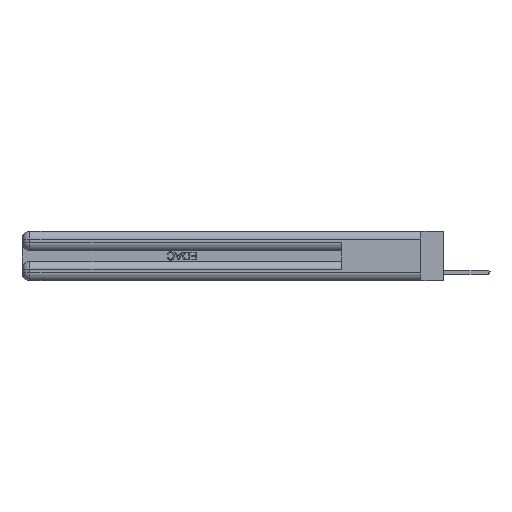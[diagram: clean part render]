
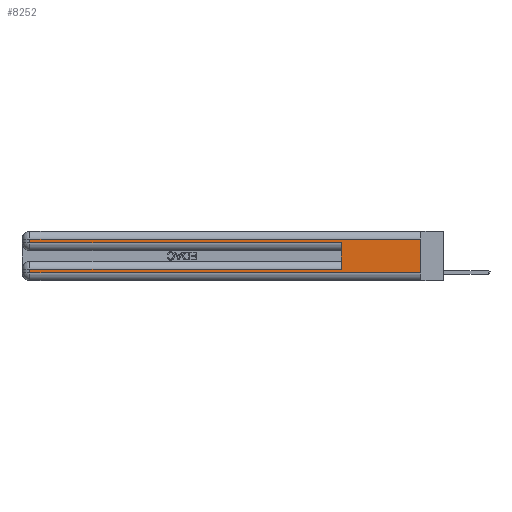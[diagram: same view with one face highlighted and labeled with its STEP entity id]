
A CAD part, left-side view. The second image highlights one B-rep face of the part: STEP entity #8252.
In plain terms, the highlighted planar face has unit normal (-1, 0, 0).
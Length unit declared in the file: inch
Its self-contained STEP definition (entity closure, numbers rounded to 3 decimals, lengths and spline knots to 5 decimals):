
#63 = VECTOR ( 'NONE', #7379, 39.37008 ) ;
#2607 = VECTOR ( 'NONE', #17444, 39.37008 ) ;
#3861 = CARTESIAN_POINT ( 'NONE',  ( 0., 0., 0.06 ) ) ;
#4646 = VECTOR ( 'NONE', #30315, 39.37008 ) ;
#4804 = DIRECTION ( 'NONE',  ( 0., 0., -1. ) ) ;
#5010 = PLANE ( 'NONE',  #29456 ) ;
#5038 = DIRECTION ( 'NONE',  ( 0., 1., 0. ) ) ;
#5150 = EDGE_LOOP ( 'NONE', ( #30249, #16295, #27626, #10470, #21544, #9117, #27784, #25649 ) ) ;
#5188 = CARTESIAN_POINT ( 'NONE',  ( 0., 0., 0.085 ) ) ;
#6665 = VERTEX_POINT ( 'NONE', #27908 ) ;
#6721 = FACE_OUTER_BOUND ( 'NONE', #5150, .T. ) ;
#7101 = CARTESIAN_POINT ( 'NONE',  ( 0., 0., 0.37 ) ) ;
#7379 = DIRECTION ( 'NONE',  ( 0., 1., 0. ) ) ;
#7549 = LINE ( 'NONE', #19179, #19463 ) ;
#7958 = EDGE_CURVE ( 'NONE', #29759, #9251, #28743, .T. ) ;
#7988 = VERTEX_POINT ( 'NONE', #22511 ) ;
#8252 = ADVANCED_FACE ( 'NONE', ( #6721 ), #5010, .F. ) ;
#8596 = CARTESIAN_POINT ( 'NONE',  ( 0., 2.94, 0.285 ) ) ;
#9117 = ORIENTED_EDGE ( 'NONE', *, *, #18526, .T. ) ;
#9251 = VERTEX_POINT ( 'NONE', #26484 ) ;
#10470 = ORIENTED_EDGE ( 'NONE', *, *, #18925, .T. ) ;
#13130 = LINE ( 'NONE', #5188, #63 ) ;
#13560 = DIRECTION ( 'NONE',  ( 0., 0., 1. ) ) ;
#13626 = CARTESIAN_POINT ( 'NONE',  ( 0., 0., 0.37 ) ) ;
#15199 = VERTEX_POINT ( 'NONE', #29937 ) ;
#15352 = DIRECTION ( 'NONE',  ( 0., 0., -1. ) ) ;
#16295 = ORIENTED_EDGE ( 'NONE', *, *, #22165, .T. ) ;
#16765 = EDGE_CURVE ( 'NONE', #27972, #24601, #7549, .T. ) ;
#16998 = CARTESIAN_POINT ( 'NONE',  ( 0., 2.94, 0.31 ) ) ;
#17180 = EDGE_CURVE ( 'NONE', #9251, #7988, #21692, .T. ) ;
#17201 = LINE ( 'NONE', #21300, #29149 ) ;
#17331 = CARTESIAN_POINT ( 'NONE',  ( 0., 2.94, 0.37 ) ) ;
#17444 = DIRECTION ( 'NONE',  ( 0., 0., -1. ) ) ;
#18526 = EDGE_CURVE ( 'NONE', #15199, #29759, #13130, .T. ) ;
#18925 = EDGE_CURVE ( 'NONE', #24601, #6665, #17201, .T. ) ;
#19179 = CARTESIAN_POINT ( 'NONE',  ( 0., 2.94, 0.37 ) ) ;
#19463 = VECTOR ( 'NONE', #15352, 39.37008 ) ;
#20529 = DIRECTION ( 'NONE',  ( 0., -1., 0. ) ) ;
#21300 = CARTESIAN_POINT ( 'NONE',  ( 0., 0., 0.285 ) ) ;
#21339 = DIRECTION ( 'NONE',  ( 1., 0., 0. ) ) ;
#21493 = DIRECTION ( 'NONE',  ( 0., -1., 0. ) ) ;
#21544 = ORIENTED_EDGE ( 'NONE', *, *, #27136, .F. ) ;
#21692 = LINE ( 'NONE', #3861, #26037 ) ;
#22165 = EDGE_CURVE ( 'NONE', #22394, #27972, #25942, .T. ) ;
#22394 = VERTEX_POINT ( 'NONE', #26722 ) ;
#22472 = CARTESIAN_POINT ( 'NONE',  ( 0., 0.6, 0.145 ) ) ;
#22507 = LINE ( 'NONE', #13626, #4646 ) ;
#22511 = CARTESIAN_POINT ( 'NONE',  ( 0., 0., 0.06 ) ) ;
#22953 = EDGE_CURVE ( 'NONE', #22394, #7988, #22507, .T. ) ;
#23674 = CARTESIAN_POINT ( 'NONE',  ( 0., 0., 0.31 ) ) ;
#23785 = VECTOR ( 'NONE', #13560, 39.37008 ) ;
#24601 = VERTEX_POINT ( 'NONE', #8596 ) ;
#25649 = ORIENTED_EDGE ( 'NONE', *, *, #17180, .T. ) ;
#25942 = LINE ( 'NONE', #23674, #28949 ) ;
#26037 = VECTOR ( 'NONE', #20529, 39.37008 ) ;
#26377 = CARTESIAN_POINT ( 'NONE',  ( 0., 2.94, 0.085 ) ) ;
#26484 = CARTESIAN_POINT ( 'NONE',  ( 0., 2.94, 0.06 ) ) ;
#26722 = CARTESIAN_POINT ( 'NONE',  ( 0., 0., 0.31 ) ) ;
#27136 = EDGE_CURVE ( 'NONE', #15199, #6665, #29059, .T. ) ;
#27626 = ORIENTED_EDGE ( 'NONE', *, *, #16765, .T. ) ;
#27784 = ORIENTED_EDGE ( 'NONE', *, *, #7958, .T. ) ;
#27908 = CARTESIAN_POINT ( 'NONE',  ( 0., 0.6, 0.285 ) ) ;
#27972 = VERTEX_POINT ( 'NONE', #16998 ) ;
#28743 = LINE ( 'NONE', #17331, #2607 ) ;
#28949 = VECTOR ( 'NONE', #5038, 39.37008 ) ;
#29059 = LINE ( 'NONE', #22472, #23785 ) ;
#29149 = VECTOR ( 'NONE', #21493, 39.37008 ) ;
#29456 = AXIS2_PLACEMENT_3D ( 'NONE', #7101, #21339, #4804 ) ;
#29759 = VERTEX_POINT ( 'NONE', #26377 ) ;
#29937 = CARTESIAN_POINT ( 'NONE',  ( 0., 0.6, 0.085 ) ) ;
#30249 = ORIENTED_EDGE ( 'NONE', *, *, #22953, .F. ) ;
#30315 = DIRECTION ( 'NONE',  ( 0., 0., -1. ) ) ;
